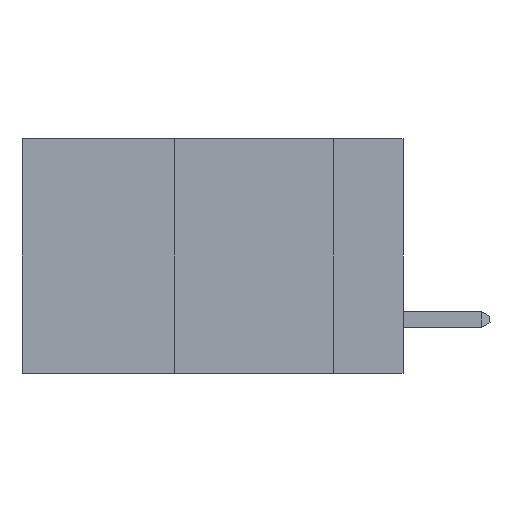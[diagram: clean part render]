
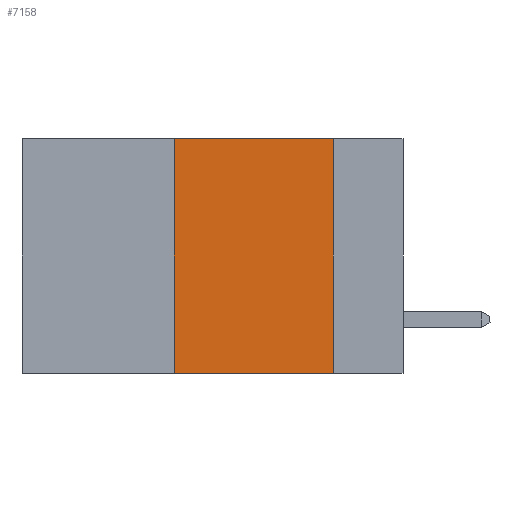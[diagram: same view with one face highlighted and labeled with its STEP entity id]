
A CAD part, left-side view. The second image highlights one B-rep face of the part: STEP entity #7158.
In plain terms, the highlighted planar face has unit normal (-1, 0, 0).
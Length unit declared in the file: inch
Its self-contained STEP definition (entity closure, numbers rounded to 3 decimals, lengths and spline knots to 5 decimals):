
#738 = VECTOR ( 'NONE', #13957, 39.37008 ) ;
#834 = PLANE ( 'NONE',  #12953 ) ;
#1650 = VECTOR ( 'NONE', #4201, 39.37008 ) ;
#1748 = EDGE_CURVE ( 'NONE', #9630, #13906, #1905, .T. ) ;
#1905 = LINE ( 'NONE', #15161, #15585 ) ;
#2152 = ORIENTED_EDGE ( 'NONE', *, *, #3908, .F. ) ;
#2249 = ORIENTED_EDGE ( 'NONE', *, *, #1748, .F. ) ;
#2849 = DIRECTION ( 'NONE',  ( 0., 0., -1. ) ) ;
#2928 = CARTESIAN_POINT ( 'NONE',  ( 0., 0.6, -0.37 ) ) ;
#3040 = EDGE_LOOP ( 'NONE', ( #7642, #2152, #2249, #15472 ) ) ;
#3058 = DIRECTION ( 'NONE',  ( 0., 0., 1. ) ) ;
#3131 = CARTESIAN_POINT ( 'NONE',  ( 0., 0.6, 0. ) ) ;
#3663 = CARTESIAN_POINT ( 'NONE',  ( 0., 0.36, 0. ) ) ;
#3908 = EDGE_CURVE ( 'NONE', #13906, #10603, #4081, .T. ) ;
#3939 = EDGE_CURVE ( 'NONE', #9630, #7437, #13628, .T. ) ;
#4081 = LINE ( 'NONE', #6808, #738 ) ;
#4201 = DIRECTION ( 'NONE',  ( 0., 0., -1. ) ) ;
#6714 = EDGE_CURVE ( 'NONE', #10603, #7437, #8703, .T. ) ;
#6808 = CARTESIAN_POINT ( 'NONE',  ( 0., 0.6, 0. ) ) ;
#7158 = ADVANCED_FACE ( 'NONE', ( #7335 ), #834, .F. ) ;
#7335 = FACE_OUTER_BOUND ( 'NONE', #3040, .T. ) ;
#7372 = CARTESIAN_POINT ( 'NONE',  ( 0., 0.36, -0.37 ) ) ;
#7437 = VERTEX_POINT ( 'NONE', #9580 ) ;
#7573 = DIRECTION ( 'NONE',  ( 1., 0., 0. ) ) ;
#7642 = ORIENTED_EDGE ( 'NONE', *, *, #6714, .F. ) ;
#8703 = LINE ( 'NONE', #10280, #1650 ) ;
#9197 = DIRECTION ( 'NONE',  ( 0., -1., 0. ) ) ;
#9580 = CARTESIAN_POINT ( 'NONE',  ( 0., 0.11, -0.37 ) ) ;
#9630 = VERTEX_POINT ( 'NONE', #7372 ) ;
#10280 = CARTESIAN_POINT ( 'NONE',  ( 0., 0.11, 0. ) ) ;
#10603 = VERTEX_POINT ( 'NONE', #13743 ) ;
#12953 = AXIS2_PLACEMENT_3D ( 'NONE', #3131, #7573, #2849 ) ;
#13628 = LINE ( 'NONE', #2928, #14961 ) ;
#13743 = CARTESIAN_POINT ( 'NONE',  ( 0., 0.11, 0. ) ) ;
#13906 = VERTEX_POINT ( 'NONE', #3663 ) ;
#13957 = DIRECTION ( 'NONE',  ( 0., -1., 0. ) ) ;
#14961 = VECTOR ( 'NONE', #9197, 39.37008 ) ;
#15161 = CARTESIAN_POINT ( 'NONE',  ( 0., 0.36, 0. ) ) ;
#15472 = ORIENTED_EDGE ( 'NONE', *, *, #3939, .T. ) ;
#15585 = VECTOR ( 'NONE', #3058, 39.37008 ) ;
